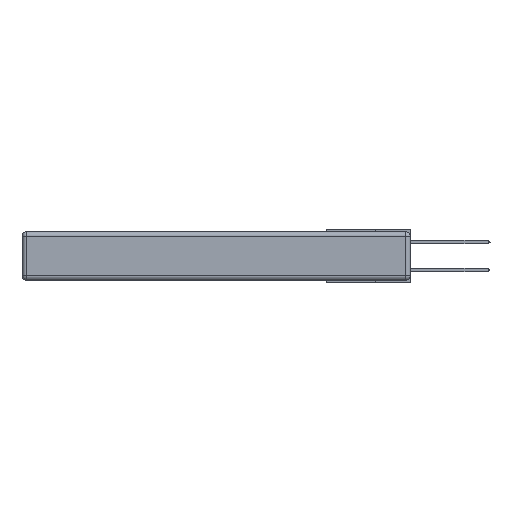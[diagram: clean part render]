
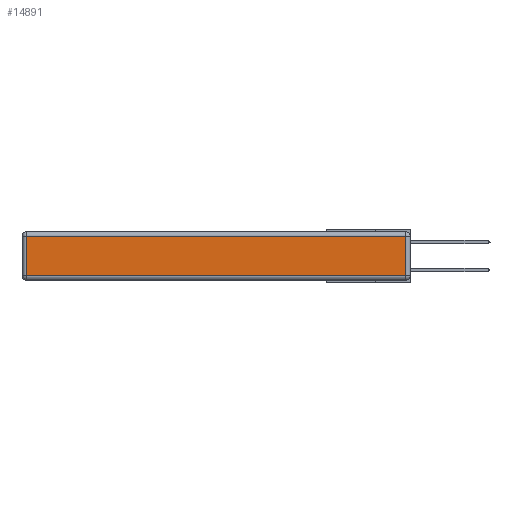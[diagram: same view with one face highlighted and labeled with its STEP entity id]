
A CAD part, left-side view. The second image highlights one B-rep face of the part: STEP entity #14891.
In plain terms, the highlighted planar face has unit normal (-1, 0, 0).
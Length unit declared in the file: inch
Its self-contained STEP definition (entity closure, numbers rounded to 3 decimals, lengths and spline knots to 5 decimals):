
#495 = ORIENTED_EDGE ( 'NONE', *, *, #5607, .T. ) ;
#1161 = PLANE ( 'NONE',  #1569 ) ;
#1431 = VERTEX_POINT ( 'NONE', #5298 ) ;
#1569 = AXIS2_PLACEMENT_3D ( 'NONE', #8228, #5627, #18459 ) ;
#3151 = DIRECTION ( 'NONE',  ( 0., 0., -1. ) ) ;
#3279 = EDGE_CURVE ( 'NONE', #18535, #1431, #8772, .T. ) ;
#4804 = LINE ( 'NONE', #14683, #17800 ) ;
#5298 = CARTESIAN_POINT ( 'NONE',  ( 0., 2.72, -0.03 ) ) ;
#5607 = EDGE_CURVE ( 'NONE', #1431, #12279, #14319, .T. ) ;
#5627 = DIRECTION ( 'NONE',  ( -1., 0., 0. ) ) ;
#5841 = EDGE_LOOP ( 'NONE', ( #17434, #15249, #7192, #495 ) ) ;
#6217 = CARTESIAN_POINT ( 'NONE',  ( 0., 2.72, -0.313 ) ) ;
#6410 = CARTESIAN_POINT ( 'NONE',  ( 0., 2.75, -0.03 ) ) ;
#6918 = CARTESIAN_POINT ( 'NONE',  ( 0., 2.72, -0.343 ) ) ;
#7192 = ORIENTED_EDGE ( 'NONE', *, *, #3279, .T. ) ;
#7472 = DIRECTION ( 'NONE',  ( 0., 0., 1. ) ) ;
#8228 = CARTESIAN_POINT ( 'NONE',  ( 0., 0., -0.343 ) ) ;
#8772 = LINE ( 'NONE', #6410, #13263 ) ;
#10543 = CARTESIAN_POINT ( 'NONE',  ( 0., 0.03, -0.03 ) ) ;
#12279 = VERTEX_POINT ( 'NONE', #6217 ) ;
#12544 = CARTESIAN_POINT ( 'NONE',  ( 0., 0.03, -0.313 ) ) ;
#12664 = VERTEX_POINT ( 'NONE', #12544 ) ;
#13263 = VECTOR ( 'NONE', #18118, 39.37008 ) ;
#13332 = VECTOR ( 'NONE', #13569, 39.37008 ) ;
#13440 = CARTESIAN_POINT ( 'NONE',  ( 0., 0., -0.313 ) ) ;
#13569 = DIRECTION ( 'NONE',  ( 0., -1., 0. ) ) ;
#13774 = LINE ( 'NONE', #13440, #13332 ) ;
#14319 = LINE ( 'NONE', #6918, #15890 ) ;
#14683 = CARTESIAN_POINT ( 'NONE',  ( 0., 0.03, -0.343 ) ) ;
#14891 = ADVANCED_FACE ( 'NONE', ( #14988 ), #1161, .T. ) ;
#14988 = FACE_OUTER_BOUND ( 'NONE', #5841, .T. ) ;
#15249 = ORIENTED_EDGE ( 'NONE', *, *, #17769, .T. ) ;
#15890 = VECTOR ( 'NONE', #3151, 39.37008 ) ;
#17262 = EDGE_CURVE ( 'NONE', #12279, #12664, #13774, .T. ) ;
#17434 = ORIENTED_EDGE ( 'NONE', *, *, #17262, .T. ) ;
#17769 = EDGE_CURVE ( 'NONE', #12664, #18535, #4804, .T. ) ;
#17800 = VECTOR ( 'NONE', #7472, 39.37008 ) ;
#18118 = DIRECTION ( 'NONE',  ( 0., 1., 0. ) ) ;
#18459 = DIRECTION ( 'NONE',  ( 0., 0., 1. ) ) ;
#18535 = VERTEX_POINT ( 'NONE', #10543 ) ;
